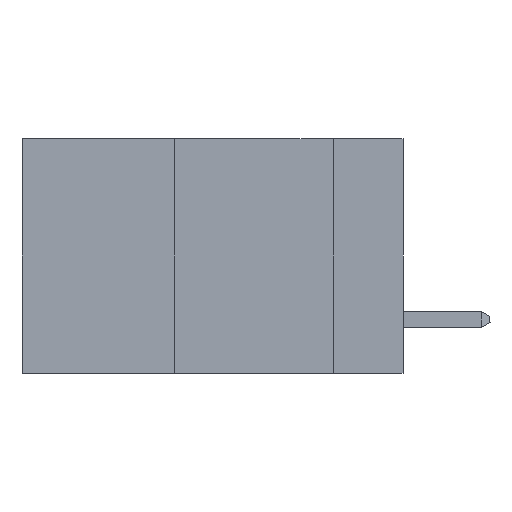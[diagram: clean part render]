
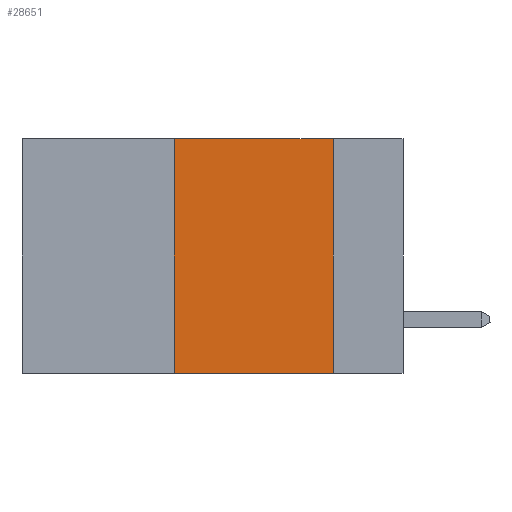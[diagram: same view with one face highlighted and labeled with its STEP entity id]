
A CAD part, left-side view. The second image highlights one B-rep face of the part: STEP entity #28651.
In plain terms, the highlighted planar face has unit normal (-1, 0, 0).
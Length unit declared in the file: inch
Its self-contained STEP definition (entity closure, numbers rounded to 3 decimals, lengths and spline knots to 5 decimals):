
#302 = ORIENTED_EDGE ( 'NONE', *, *, #1538, .F. ) ;
#446 = VERTEX_POINT ( 'NONE', #6570 ) ;
#645 = VERTEX_POINT ( 'NONE', #16541 ) ;
#658 = CARTESIAN_POINT ( 'NONE',  ( 0., 0.36, 0. ) ) ;
#667 = VECTOR ( 'NONE', #9268, 39.37008 ) ;
#1072 = CARTESIAN_POINT ( 'NONE',  ( 0., 0.11, 0. ) ) ;
#1298 = VERTEX_POINT ( 'NONE', #16986 ) ;
#1538 = EDGE_CURVE ( 'NONE', #645, #1298, #29101, .T. ) ;
#2798 = DIRECTION ( 'NONE',  ( 0., -1., 0. ) ) ;
#4210 = ORIENTED_EDGE ( 'NONE', *, *, #5208, .F. ) ;
#4270 = EDGE_LOOP ( 'NONE', ( #4210, #9495, #302, #14647 ) ) ;
#4998 = CARTESIAN_POINT ( 'NONE',  ( 0., 0.11, -0.37 ) ) ;
#5208 = EDGE_CURVE ( 'NONE', #446, #14118, #12205, .T. ) ;
#6570 = CARTESIAN_POINT ( 'NONE',  ( 0., 0.11, 0. ) ) ;
#7275 = DIRECTION ( 'NONE',  ( 1., 0., 0. ) ) ;
#8523 = VECTOR ( 'NONE', #2798, 39.37008 ) ;
#9268 = DIRECTION ( 'NONE',  ( 0., -1., 0. ) ) ;
#9495 = ORIENTED_EDGE ( 'NONE', *, *, #15457, .F. ) ;
#11355 = VECTOR ( 'NONE', #16476, 39.37008 ) ;
#12205 = LINE ( 'NONE', #1072, #11355 ) ;
#14118 = VERTEX_POINT ( 'NONE', #4998 ) ;
#14647 = ORIENTED_EDGE ( 'NONE', *, *, #29431, .T. ) ;
#14768 = FACE_OUTER_BOUND ( 'NONE', #4270, .T. ) ;
#15457 = EDGE_CURVE ( 'NONE', #1298, #446, #32906, .T. ) ;
#16476 = DIRECTION ( 'NONE',  ( 0., 0., -1. ) ) ;
#16541 = CARTESIAN_POINT ( 'NONE',  ( 0., 0.36, -0.37 ) ) ;
#16986 = CARTESIAN_POINT ( 'NONE',  ( 0., 0.36, 0. ) ) ;
#17300 = CARTESIAN_POINT ( 'NONE',  ( 0., 0.6, 0. ) ) ;
#17965 = LINE ( 'NONE', #26251, #8523 ) ;
#19134 = AXIS2_PLACEMENT_3D ( 'NONE', #25848, #7275, #28395 ) ;
#22676 = PLANE ( 'NONE',  #19134 ) ;
#24533 = VECTOR ( 'NONE', #32411, 39.37008 ) ;
#25848 = CARTESIAN_POINT ( 'NONE',  ( 0., 0.6, 0. ) ) ;
#26251 = CARTESIAN_POINT ( 'NONE',  ( 0., 0.6, -0.37 ) ) ;
#28395 = DIRECTION ( 'NONE',  ( 0., 0., -1. ) ) ;
#28651 = ADVANCED_FACE ( 'NONE', ( #14768 ), #22676, .F. ) ;
#29101 = LINE ( 'NONE', #658, #24533 ) ;
#29431 = EDGE_CURVE ( 'NONE', #645, #14118, #17965, .T. ) ;
#32411 = DIRECTION ( 'NONE',  ( 0., 0., 1. ) ) ;
#32906 = LINE ( 'NONE', #17300, #667 ) ;
